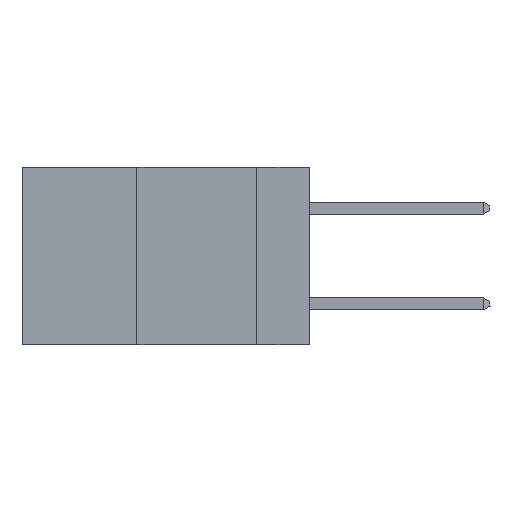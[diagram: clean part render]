
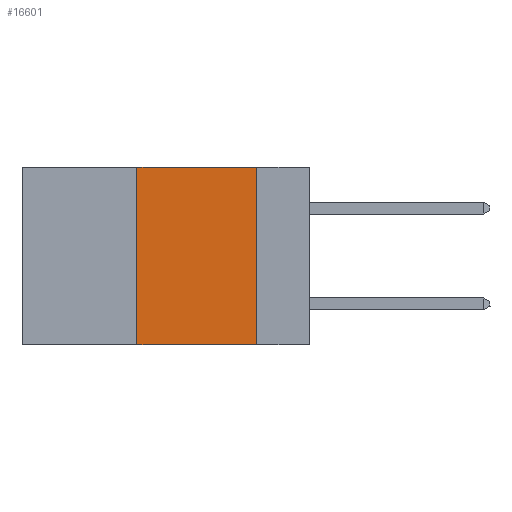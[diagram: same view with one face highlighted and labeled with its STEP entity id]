
A CAD part, left-side view. The second image highlights one B-rep face of the part: STEP entity #16601.
In plain terms, the highlighted planar face has unit normal (-1, 0, 0).
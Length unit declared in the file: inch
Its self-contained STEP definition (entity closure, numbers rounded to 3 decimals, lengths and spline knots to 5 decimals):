
#436 = CARTESIAN_POINT ( 'NONE',  ( 0., 0.6, -0.37 ) ) ;
#1594 = LINE ( 'NONE', #12451, #6575 ) ;
#2978 = VERTEX_POINT ( 'NONE', #11214 ) ;
#3376 = DIRECTION ( 'NONE',  ( 0., 0., 1. ) ) ;
#3680 = LINE ( 'NONE', #5622, #10934 ) ;
#4326 = ORIENTED_EDGE ( 'NONE', *, *, #11202, .F. ) ;
#5068 = CARTESIAN_POINT ( 'NONE',  ( 0., 0.36, 0. ) ) ;
#5622 = CARTESIAN_POINT ( 'NONE',  ( 0., 0.11, 0. ) ) ;
#5828 = VERTEX_POINT ( 'NONE', #17911 ) ;
#6575 = VECTOR ( 'NONE', #10520, 39.37008 ) ;
#9604 = LINE ( 'NONE', #436, #20807 ) ;
#10520 = DIRECTION ( 'NONE',  ( 0., -1., 0. ) ) ;
#10648 = EDGE_CURVE ( 'NONE', #15049, #14704, #9604, .T. ) ;
#10934 = VECTOR ( 'NONE', #20524, 39.37008 ) ;
#11202 = EDGE_CURVE ( 'NONE', #15049, #5828, #16105, .T. ) ;
#11214 = CARTESIAN_POINT ( 'NONE',  ( 0., 0.11, 0. ) ) ;
#11365 = AXIS2_PLACEMENT_3D ( 'NONE', #23335, #18116, #21497 ) ;
#11883 = CARTESIAN_POINT ( 'NONE',  ( 0., 0.11, -0.37 ) ) ;
#11968 = ORIENTED_EDGE ( 'NONE', *, *, #13095, .F. ) ;
#12085 = CARTESIAN_POINT ( 'NONE',  ( 0., 0.36, -0.37 ) ) ;
#12451 = CARTESIAN_POINT ( 'NONE',  ( 0., 0.6, 0. ) ) ;
#13095 = EDGE_CURVE ( 'NONE', #2978, #14704, #3680, .T. ) ;
#14704 = VERTEX_POINT ( 'NONE', #11883 ) ;
#15049 = VERTEX_POINT ( 'NONE', #12085 ) ;
#15914 = EDGE_LOOP ( 'NONE', ( #11968, #23544, #4326, #22175 ) ) ;
#16105 = LINE ( 'NONE', #5068, #23547 ) ;
#16320 = FACE_OUTER_BOUND ( 'NONE', #15914, .T. ) ;
#16601 = ADVANCED_FACE ( 'NONE', ( #16320 ), #21617, .F. ) ;
#17017 = DIRECTION ( 'NONE',  ( 0., -1., 0. ) ) ;
#17911 = CARTESIAN_POINT ( 'NONE',  ( 0., 0.36, 0. ) ) ;
#18116 = DIRECTION ( 'NONE',  ( 1., 0., 0. ) ) ;
#20524 = DIRECTION ( 'NONE',  ( 0., 0., -1. ) ) ;
#20807 = VECTOR ( 'NONE', #17017, 39.37008 ) ;
#21497 = DIRECTION ( 'NONE',  ( 0., 0., -1. ) ) ;
#21617 = PLANE ( 'NONE',  #11365 ) ;
#22175 = ORIENTED_EDGE ( 'NONE', *, *, #10648, .T. ) ;
#22317 = EDGE_CURVE ( 'NONE', #5828, #2978, #1594, .T. ) ;
#23335 = CARTESIAN_POINT ( 'NONE',  ( 0., 0.6, 0. ) ) ;
#23544 = ORIENTED_EDGE ( 'NONE', *, *, #22317, .F. ) ;
#23547 = VECTOR ( 'NONE', #3376, 39.37008 ) ;
